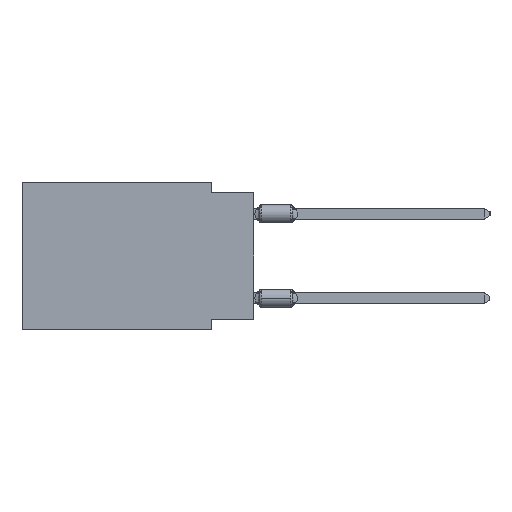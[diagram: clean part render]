
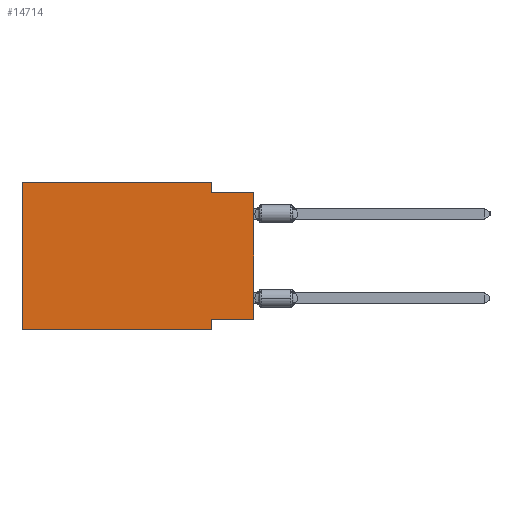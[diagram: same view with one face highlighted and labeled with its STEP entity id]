
A CAD part, left-side view. The second image highlights one B-rep face of the part: STEP entity #14714.
In plain terms, the highlighted planar face has unit normal (-1, 0, 0).
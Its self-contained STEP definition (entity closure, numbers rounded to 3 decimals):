
#112 = EDGE_LOOP ( 'NONE', ( #1732, #5777, #30447, #21216, #8784, #13271, #27169, #21760 ) ) ;
#398 = EDGE_CURVE ( 'NONE', #14484, #34950, #26417, .T. ) ;
#606 = AXIS2_PLACEMENT_3D ( 'NONE', #16713, #32284, #17412 ) ;
#1552 = CARTESIAN_POINT ( 'NONE',  ( 0., 0., -0.635 ) ) ;
#1732 = ORIENTED_EDGE ( 'NONE', *, *, #21277, .T. ) ;
#2612 = VERTEX_POINT ( 'NONE', #4042 ) ;
#2873 = EDGE_CURVE ( 'NONE', #19632, #14484, #26255, .T. ) ;
#2955 = DIRECTION ( 'NONE',  ( 0., -1., 0. ) ) ;
#3619 = CARTESIAN_POINT ( 'NONE',  ( 0., 13.97, 0. ) ) ;
#4042 = CARTESIAN_POINT ( 'NONE',  ( 0., 0., -0.635 ) ) ;
#5748 = CARTESIAN_POINT ( 'NONE',  ( 0., 2.54, -8.255 ) ) ;
#5777 = ORIENTED_EDGE ( 'NONE', *, *, #29582, .F. ) ;
#5779 = LINE ( 'NONE', #11441, #9392 ) ;
#7486 = VECTOR ( 'NONE', #29283, 1000. ) ;
#8217 = VECTOR ( 'NONE', #25123, 1000. ) ;
#8769 = VECTOR ( 'NONE', #32360, 1000. ) ;
#8784 = ORIENTED_EDGE ( 'NONE', *, *, #2873, .F. ) ;
#8965 = EDGE_CURVE ( 'NONE', #19811, #23768, #11994, .T. ) ;
#9392 = VECTOR ( 'NONE', #2955, 1000. ) ;
#9997 = VECTOR ( 'NONE', #10740, 1000. ) ;
#10740 = DIRECTION ( 'NONE',  ( 0., 0., -1. ) ) ;
#11441 = CARTESIAN_POINT ( 'NONE',  ( 0., 13.97, -8.89 ) ) ;
#11994 = LINE ( 'NONE', #29731, #34530 ) ;
#13271 = ORIENTED_EDGE ( 'NONE', *, *, #33295, .T. ) ;
#13447 = LINE ( 'NONE', #36447, #21677 ) ;
#13605 = LINE ( 'NONE', #1552, #8217 ) ;
#14484 = VERTEX_POINT ( 'NONE', #18071 ) ;
#14714 = ADVANCED_FACE ( 'NONE', ( #19551 ), #36698, .F. ) ;
#14811 = CARTESIAN_POINT ( 'NONE',  ( 0., 0., -8.255 ) ) ;
#16713 = CARTESIAN_POINT ( 'NONE',  ( 0., 13.97, 0. ) ) ;
#17412 = DIRECTION ( 'NONE',  ( 0., 0., -1. ) ) ;
#17519 = VERTEX_POINT ( 'NONE', #36931 ) ;
#17944 = DIRECTION ( 'NONE',  ( 0., -1., 0. ) ) ;
#18071 = CARTESIAN_POINT ( 'NONE',  ( 0., 13.97, 0. ) ) ;
#18398 = VERTEX_POINT ( 'NONE', #33813 ) ;
#19551 = FACE_OUTER_BOUND ( 'NONE', #112, .T. ) ;
#19632 = VERTEX_POINT ( 'NONE', #28041 ) ;
#19811 = VERTEX_POINT ( 'NONE', #5748 ) ;
#21216 = ORIENTED_EDGE ( 'NONE', *, *, #398, .F. ) ;
#21277 = EDGE_CURVE ( 'NONE', #17519, #2612, #13447, .T. ) ;
#21677 = VECTOR ( 'NONE', #35904, 1000. ) ;
#21760 = ORIENTED_EDGE ( 'NONE', *, *, #28903, .F. ) ;
#23768 = VERTEX_POINT ( 'NONE', #31476 ) ;
#24036 = LINE ( 'NONE', #35334, #9997 ) ;
#24766 = EDGE_CURVE ( 'NONE', #34950, #18398, #24036, .T. ) ;
#25123 = DIRECTION ( 'NONE',  ( 0., -1., 0. ) ) ;
#26224 = CARTESIAN_POINT ( 'NONE',  ( 0., 13.97, 0. ) ) ;
#26255 = LINE ( 'NONE', #3619, #7486 ) ;
#26417 = LINE ( 'NONE', #26224, #30253 ) ;
#27169 = ORIENTED_EDGE ( 'NONE', *, *, #8965, .F. ) ;
#28041 = CARTESIAN_POINT ( 'NONE',  ( 0., 13.97, -8.89 ) ) ;
#28903 = EDGE_CURVE ( 'NONE', #17519, #19811, #35179, .T. ) ;
#29283 = DIRECTION ( 'NONE',  ( 0., 0., 1. ) ) ;
#29582 = EDGE_CURVE ( 'NONE', #18398, #2612, #13605, .T. ) ;
#29731 = CARTESIAN_POINT ( 'NONE',  ( 0., 2.54, -8.89 ) ) ;
#30253 = VECTOR ( 'NONE', #17944, 1000. ) ;
#30447 = ORIENTED_EDGE ( 'NONE', *, *, #24766, .F. ) ;
#31037 = CARTESIAN_POINT ( 'NONE',  ( 0., 2.54, 0. ) ) ;
#31476 = CARTESIAN_POINT ( 'NONE',  ( 0., 2.54, -8.89 ) ) ;
#32284 = DIRECTION ( 'NONE',  ( 1., 0., 0. ) ) ;
#32360 = DIRECTION ( 'NONE',  ( 0., 1., 0. ) ) ;
#33295 = EDGE_CURVE ( 'NONE', #19632, #23768, #5779, .T. ) ;
#33813 = CARTESIAN_POINT ( 'NONE',  ( 0., 2.54, -0.635 ) ) ;
#34530 = VECTOR ( 'NONE', #35380, 1000. ) ;
#34950 = VERTEX_POINT ( 'NONE', #31037 ) ;
#35179 = LINE ( 'NONE', #14811, #8769 ) ;
#35334 = CARTESIAN_POINT ( 'NONE',  ( 0., 2.54, 0. ) ) ;
#35380 = DIRECTION ( 'NONE',  ( 0., 0., -1. ) ) ;
#35904 = DIRECTION ( 'NONE',  ( 0., 0., 1. ) ) ;
#36447 = CARTESIAN_POINT ( 'NONE',  ( 0., 0., 0. ) ) ;
#36698 = PLANE ( 'NONE',  #606 ) ;
#36931 = CARTESIAN_POINT ( 'NONE',  ( 0., 0., -8.255 ) ) ;
